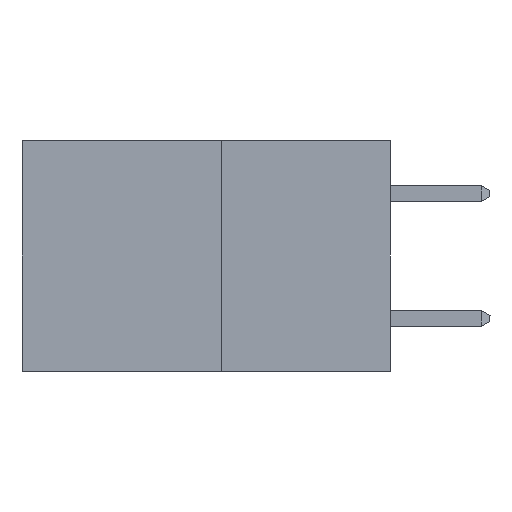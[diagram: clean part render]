
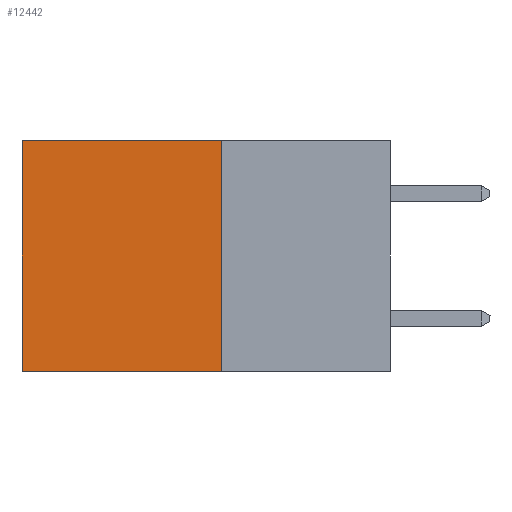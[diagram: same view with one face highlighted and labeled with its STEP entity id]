
A CAD part, left-side view. The second image highlights one B-rep face of the part: STEP entity #12442.
In plain terms, the highlighted planar face has unit normal (-1, 0, 0).
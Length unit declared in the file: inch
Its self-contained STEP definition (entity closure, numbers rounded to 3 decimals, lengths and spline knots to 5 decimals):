
#4 = EDGE_LOOP ( 'NONE', ( #874, #7779, #9168, #4485 ) ) ;
#874 = ORIENTED_EDGE ( 'NONE', *, *, #4863, .T. ) ;
#1856 = CARTESIAN_POINT ( 'NONE',  ( 0.277, 0.27, 0. ) ) ;
#2773 = CARTESIAN_POINT ( 'NONE',  ( 0.277, 0.27, -0.37 ) ) ;
#2930 = DIRECTION ( 'NONE',  ( 0., 1., 0. ) ) ;
#2955 = VERTEX_POINT ( 'NONE', #5411 ) ;
#4485 = ORIENTED_EDGE ( 'NONE', *, *, #10915, .T. ) ;
#4532 = PLANE ( 'NONE',  #6422 ) ;
#4537 = EDGE_CURVE ( 'NONE', #9032, #9279, #10759, .T. ) ;
#4581 = CARTESIAN_POINT ( 'NONE',  ( 0.277, 0.27, -0.37 ) ) ;
#4863 = EDGE_CURVE ( 'NONE', #10294, #2955, #10008, .T. ) ;
#4995 = CARTESIAN_POINT ( 'NONE',  ( 0.277, 0.27, -0.37 ) ) ;
#5411 = CARTESIAN_POINT ( 'NONE',  ( 0.277, 0.59, -0.37 ) ) ;
#5613 = DIRECTION ( 'NONE',  ( 1., 0., 0. ) ) ;
#6422 = AXIS2_PLACEMENT_3D ( 'NONE', #4581, #5613, #12473 ) ;
#7779 = ORIENTED_EDGE ( 'NONE', *, *, #8685, .F. ) ;
#8092 = LINE ( 'NONE', #1856, #12945 ) ;
#8241 = DIRECTION ( 'NONE',  ( 0., 0., -1. ) ) ;
#8685 = EDGE_CURVE ( 'NONE', #9279, #2955, #9528, .T. ) ;
#9032 = VERTEX_POINT ( 'NONE', #10476 ) ;
#9168 = ORIENTED_EDGE ( 'NONE', *, *, #4537, .F. ) ;
#9279 = VERTEX_POINT ( 'NONE', #2773 ) ;
#9528 = LINE ( 'NONE', #4995, #11470 ) ;
#9709 = VECTOR ( 'NONE', #12587, 39.37008 ) ;
#9906 = FACE_OUTER_BOUND ( 'NONE', #4, .T. ) ;
#10008 = LINE ( 'NONE', #10662, #9709 ) ;
#10294 = VERTEX_POINT ( 'NONE', #11028 ) ;
#10458 = VECTOR ( 'NONE', #8241, 39.37008 ) ;
#10476 = CARTESIAN_POINT ( 'NONE',  ( 0.277, 0.27, 0. ) ) ;
#10662 = CARTESIAN_POINT ( 'NONE',  ( 0.277, 0.59, -0.37 ) ) ;
#10759 = LINE ( 'NONE', #12118, #10458 ) ;
#10915 = EDGE_CURVE ( 'NONE', #9032, #10294, #8092, .T. ) ;
#11028 = CARTESIAN_POINT ( 'NONE',  ( 0.277, 0.59, 0. ) ) ;
#11470 = VECTOR ( 'NONE', #12882, 39.37008 ) ;
#12118 = CARTESIAN_POINT ( 'NONE',  ( 0.277, 0.27, -0.37 ) ) ;
#12442 = ADVANCED_FACE ( 'NONE', ( #9906 ), #4532, .F. ) ;
#12473 = DIRECTION ( 'NONE',  ( 0., 0., -1. ) ) ;
#12587 = DIRECTION ( 'NONE',  ( 0., 0., -1. ) ) ;
#12882 = DIRECTION ( 'NONE',  ( 0., 1., 0. ) ) ;
#12945 = VECTOR ( 'NONE', #2930, 39.37008 ) ;
